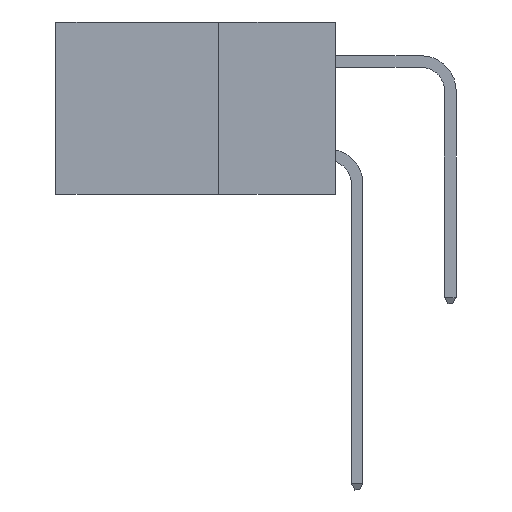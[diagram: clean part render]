
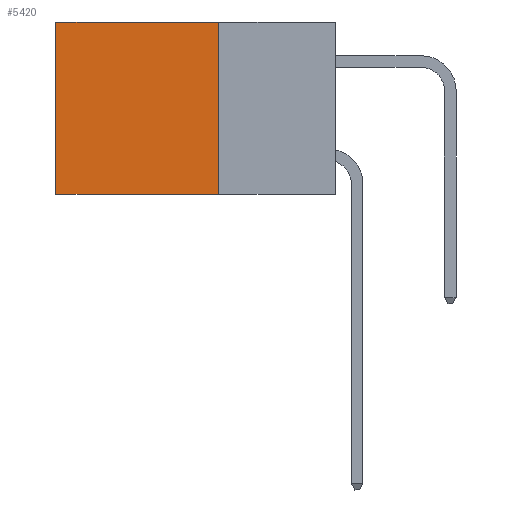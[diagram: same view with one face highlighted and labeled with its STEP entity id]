
A CAD part, left-side view. The second image highlights one B-rep face of the part: STEP entity #5420.
In plain terms, the highlighted planar face has unit normal (-1, 0, 0).
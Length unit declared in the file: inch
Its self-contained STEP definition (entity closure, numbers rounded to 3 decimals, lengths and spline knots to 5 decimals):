
#123 = EDGE_CURVE ( 'NONE', #329, #4079, #1994, .T. ) ;
#246 = CARTESIAN_POINT ( 'NONE',  ( 0.2875, 0.25, 0. ) ) ;
#317 = CARTESIAN_POINT ( 'NONE',  ( 0.2875, 0.6, -0.37 ) ) ;
#329 = VERTEX_POINT ( 'NONE', #5891 ) ;
#352 = EDGE_CURVE ( 'NONE', #4944, #4079, #9645, .T. ) ;
#375 = DIRECTION ( 'NONE',  ( 0., 0., -1. ) ) ;
#717 = AXIS2_PLACEMENT_3D ( 'NONE', #13774, #7217, #375 ) ;
#1730 = FACE_OUTER_BOUND ( 'NONE', #12269, .T. ) ;
#1905 = ORIENTED_EDGE ( 'NONE', *, *, #4917, .F. ) ;
#1994 = LINE ( 'NONE', #7445, #4336 ) ;
#2542 = VERTEX_POINT ( 'NONE', #246 ) ;
#4079 = VERTEX_POINT ( 'NONE', #317 ) ;
#4119 = CARTESIAN_POINT ( 'NONE',  ( 0.2875, 0.25, -0.37 ) ) ;
#4336 = VECTOR ( 'NONE', #7408, 39.37008 ) ;
#4917 = EDGE_CURVE ( 'NONE', #2542, #4944, #5546, .T. ) ;
#4944 = VERTEX_POINT ( 'NONE', #4119 ) ;
#4951 = PLANE ( 'NONE',  #717 ) ;
#5218 = CARTESIAN_POINT ( 'NONE',  ( 0.2875, 0.25, 0. ) ) ;
#5420 = ADVANCED_FACE ( 'NONE', ( #1730 ), #4951, .F. ) ;
#5468 = DIRECTION ( 'NONE',  ( 0., 1., 0. ) ) ;
#5490 = CARTESIAN_POINT ( 'NONE',  ( 0.2875, 0.25, -0.37 ) ) ;
#5546 = LINE ( 'NONE', #5218, #11404 ) ;
#5891 = CARTESIAN_POINT ( 'NONE',  ( 0.2875, 0.6, 0. ) ) ;
#7217 = DIRECTION ( 'NONE',  ( 1., 0., 0. ) ) ;
#7408 = DIRECTION ( 'NONE',  ( 0., 0., -1. ) ) ;
#7445 = CARTESIAN_POINT ( 'NONE',  ( 0.2875, 0.6, 0. ) ) ;
#7496 = DIRECTION ( 'NONE',  ( 0., 1., 0. ) ) ;
#9645 = LINE ( 'NONE', #5490, #9989 ) ;
#9989 = VECTOR ( 'NONE', #5468, 39.37008 ) ;
#10270 = EDGE_CURVE ( 'NONE', #2542, #329, #11565, .T. ) ;
#10896 = ORIENTED_EDGE ( 'NONE', *, *, #10270, .T. ) ;
#11404 = VECTOR ( 'NONE', #12926, 39.37008 ) ;
#11565 = LINE ( 'NONE', #12944, #14122 ) ;
#12269 = EDGE_LOOP ( 'NONE', ( #13387, #13199, #1905, #10896 ) ) ;
#12926 = DIRECTION ( 'NONE',  ( 0., 0., -1. ) ) ;
#12944 = CARTESIAN_POINT ( 'NONE',  ( 0.2875, 0.25, 0. ) ) ;
#13199 = ORIENTED_EDGE ( 'NONE', *, *, #352, .F. ) ;
#13387 = ORIENTED_EDGE ( 'NONE', *, *, #123, .T. ) ;
#13774 = CARTESIAN_POINT ( 'NONE',  ( 0.2875, 0.25, 0. ) ) ;
#14122 = VECTOR ( 'NONE', #7496, 39.37008 ) ;
